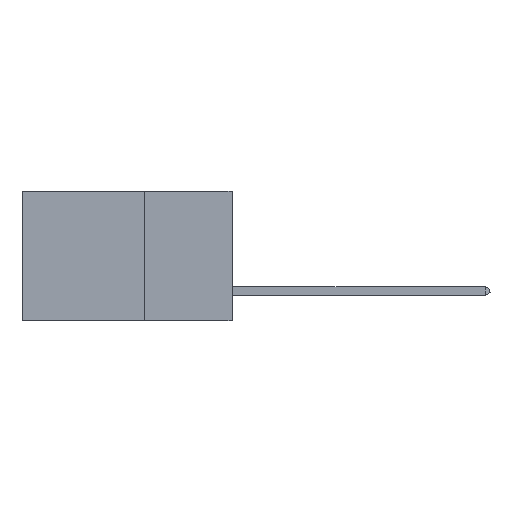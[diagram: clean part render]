
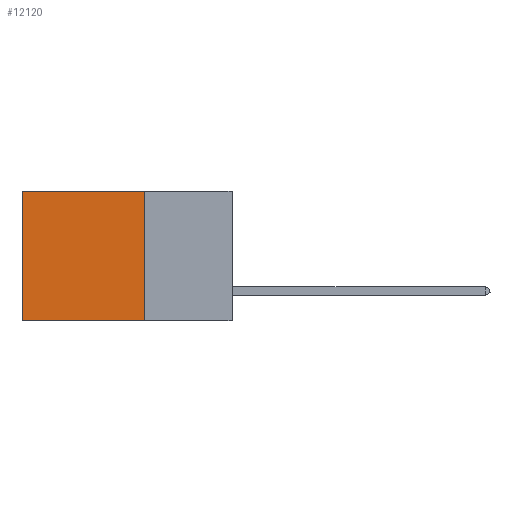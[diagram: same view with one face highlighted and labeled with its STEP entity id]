
A CAD part, left-side view. The second image highlights one B-rep face of the part: STEP entity #12120.
In plain terms, the highlighted planar face has unit normal (-1, 0, 0).
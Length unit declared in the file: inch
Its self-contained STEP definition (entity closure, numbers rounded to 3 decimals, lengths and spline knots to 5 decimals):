
#38 = VECTOR ( 'NONE', #19145, 39.37008 ) ;
#649 = DIRECTION ( 'NONE',  ( 0., 0., -1. ) ) ;
#950 = VECTOR ( 'NONE', #12643, 39.37008 ) ;
#1909 = LINE ( 'NONE', #6431, #17269 ) ;
#2068 = CARTESIAN_POINT ( 'NONE',  ( 0.2875, 0.25, -0.37 ) ) ;
#2467 = ORIENTED_EDGE ( 'NONE', *, *, #18333, .F. ) ;
#3654 = LINE ( 'NONE', #7500, #38 ) ;
#3937 = AXIS2_PLACEMENT_3D ( 'NONE', #10621, #7141, #649 ) ;
#4179 = CARTESIAN_POINT ( 'NONE',  ( 0.2875, 0.25, 0. ) ) ;
#4637 = CARTESIAN_POINT ( 'NONE',  ( 0.2875, 0.6, 0. ) ) ;
#4656 = EDGE_CURVE ( 'NONE', #20990, #10042, #14309, .T. ) ;
#5419 = PLANE ( 'NONE',  #3937 ) ;
#6431 = CARTESIAN_POINT ( 'NONE',  ( 0.2875, 0.25, -0.37 ) ) ;
#7141 = DIRECTION ( 'NONE',  ( 1., 0., 0. ) ) ;
#7315 = EDGE_CURVE ( 'NONE', #13746, #8040, #3654, .T. ) ;
#7500 = CARTESIAN_POINT ( 'NONE',  ( 0.2875, 0.6, 0. ) ) ;
#8040 = VERTEX_POINT ( 'NONE', #14788 ) ;
#8594 = ORIENTED_EDGE ( 'NONE', *, *, #7315, .T. ) ;
#8760 = LINE ( 'NONE', #4179, #950 ) ;
#8956 = DIRECTION ( 'NONE',  ( 0., 0., -1. ) ) ;
#10042 = VERTEX_POINT ( 'NONE', #2068 ) ;
#10621 = CARTESIAN_POINT ( 'NONE',  ( 0.2875, 0.25, 0. ) ) ;
#10703 = VECTOR ( 'NONE', #8956, 39.37008 ) ;
#12120 = ADVANCED_FACE ( 'NONE', ( #15060 ), #5419, .F. ) ;
#12643 = DIRECTION ( 'NONE',  ( 0., 1., 0. ) ) ;
#13017 = CARTESIAN_POINT ( 'NONE',  ( 0.2875, 0.25, 0. ) ) ;
#13119 = DIRECTION ( 'NONE',  ( 0., 1., 0. ) ) ;
#13746 = VERTEX_POINT ( 'NONE', #4637 ) ;
#13994 = CARTESIAN_POINT ( 'NONE',  ( 0.2875, 0.25, 0. ) ) ;
#14309 = LINE ( 'NONE', #13994, #10703 ) ;
#14743 = EDGE_CURVE ( 'NONE', #20990, #13746, #8760, .T. ) ;
#14788 = CARTESIAN_POINT ( 'NONE',  ( 0.2875, 0.6, -0.37 ) ) ;
#15060 = FACE_OUTER_BOUND ( 'NONE', #17948, .T. ) ;
#15064 = ORIENTED_EDGE ( 'NONE', *, *, #14743, .T. ) ;
#17269 = VECTOR ( 'NONE', #13119, 39.37008 ) ;
#17948 = EDGE_LOOP ( 'NONE', ( #8594, #2467, #19085, #15064 ) ) ;
#18333 = EDGE_CURVE ( 'NONE', #10042, #8040, #1909, .T. ) ;
#19085 = ORIENTED_EDGE ( 'NONE', *, *, #4656, .F. ) ;
#19145 = DIRECTION ( 'NONE',  ( 0., 0., -1. ) ) ;
#20990 = VERTEX_POINT ( 'NONE', #13017 ) ;
